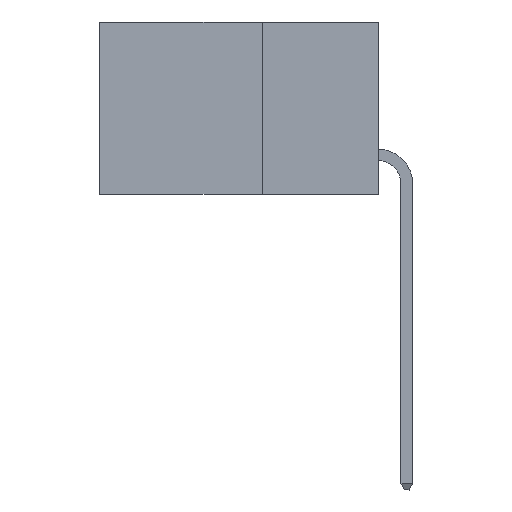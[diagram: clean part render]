
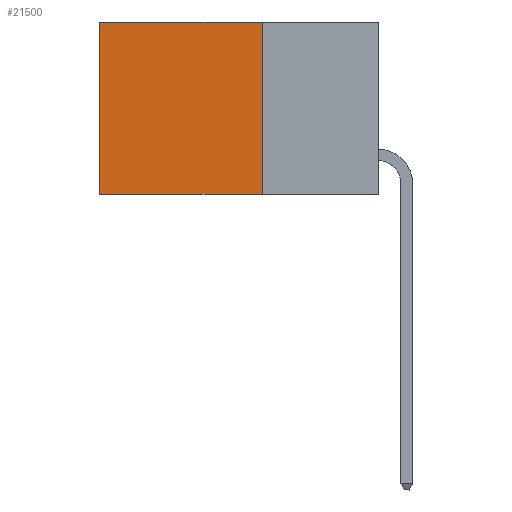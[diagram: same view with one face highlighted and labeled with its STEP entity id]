
A CAD part, left-side view. The second image highlights one B-rep face of the part: STEP entity #21500.
In plain terms, the highlighted planar face has unit normal (-1, 0, 0).
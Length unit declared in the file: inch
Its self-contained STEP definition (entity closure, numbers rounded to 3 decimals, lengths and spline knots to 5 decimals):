
#1852 = CARTESIAN_POINT ( 'NONE',  ( 0.298, 0.6, 0. ) ) ;
#2404 = EDGE_LOOP ( 'NONE', ( #28049, #20697, #15978, #25154 ) ) ;
#2917 = VERTEX_POINT ( 'NONE', #28368 ) ;
#4335 = DIRECTION ( 'NONE',  ( 0., 0., -1. ) ) ;
#4535 = LINE ( 'NONE', #16215, #21635 ) ;
#9197 = EDGE_CURVE ( 'NONE', #28325, #10315, #27255, .T. ) ;
#10315 = VERTEX_POINT ( 'NONE', #23925 ) ;
#10473 = VERTEX_POINT ( 'NONE', #26710 ) ;
#12213 = DIRECTION ( 'NONE',  ( 1., 0., 0. ) ) ;
#12951 = EDGE_CURVE ( 'NONE', #10473, #2917, #4535, .T. ) ;
#13142 = EDGE_CURVE ( 'NONE', #2917, #10315, #22364, .T. ) ;
#13489 = FACE_OUTER_BOUND ( 'NONE', #2404, .T. ) ;
#13517 = LINE ( 'NONE', #26160, #24582 ) ;
#14006 = DIRECTION ( 'NONE',  ( 0., 0., -1. ) ) ;
#15978 = ORIENTED_EDGE ( 'NONE', *, *, #12951, .F. ) ;
#16215 = CARTESIAN_POINT ( 'NONE',  ( 0.298, 0.25, 0. ) ) ;
#17146 = VECTOR ( 'NONE', #19742, 39.37008 ) ;
#18857 = PLANE ( 'NONE',  #24558 ) ;
#19742 = DIRECTION ( 'NONE',  ( 0., 1., 0. ) ) ;
#20697 = ORIENTED_EDGE ( 'NONE', *, *, #13142, .F. ) ;
#21050 = EDGE_CURVE ( 'NONE', #10473, #28325, #13517, .T. ) ;
#21435 = VECTOR ( 'NONE', #4335, 39.37008 ) ;
#21500 = ADVANCED_FACE ( 'NONE', ( #13489 ), #18857, .F. ) ;
#21635 = VECTOR ( 'NONE', #14006, 39.37008 ) ;
#21859 = CARTESIAN_POINT ( 'NONE',  ( 0.298, 0.25, -0.37 ) ) ;
#22364 = LINE ( 'NONE', #21859, #17146 ) ;
#23269 = CARTESIAN_POINT ( 'NONE',  ( 0.298, 0.25, 0. ) ) ;
#23925 = CARTESIAN_POINT ( 'NONE',  ( 0.298, 0.6, -0.37 ) ) ;
#24275 = CARTESIAN_POINT ( 'NONE',  ( 0.298, 0.6, 0. ) ) ;
#24558 = AXIS2_PLACEMENT_3D ( 'NONE', #23269, #12213, #27659 ) ;
#24582 = VECTOR ( 'NONE', #28361, 39.37008 ) ;
#25154 = ORIENTED_EDGE ( 'NONE', *, *, #21050, .T. ) ;
#26160 = CARTESIAN_POINT ( 'NONE',  ( 0.298, 0.25, 0. ) ) ;
#26710 = CARTESIAN_POINT ( 'NONE',  ( 0.298, 0.25, 0. ) ) ;
#27255 = LINE ( 'NONE', #24275, #21435 ) ;
#27659 = DIRECTION ( 'NONE',  ( 0., 0., -1. ) ) ;
#28049 = ORIENTED_EDGE ( 'NONE', *, *, #9197, .T. ) ;
#28325 = VERTEX_POINT ( 'NONE', #1852 ) ;
#28361 = DIRECTION ( 'NONE',  ( 0., 1., 0. ) ) ;
#28368 = CARTESIAN_POINT ( 'NONE',  ( 0.298, 0.25, -0.37 ) ) ;
